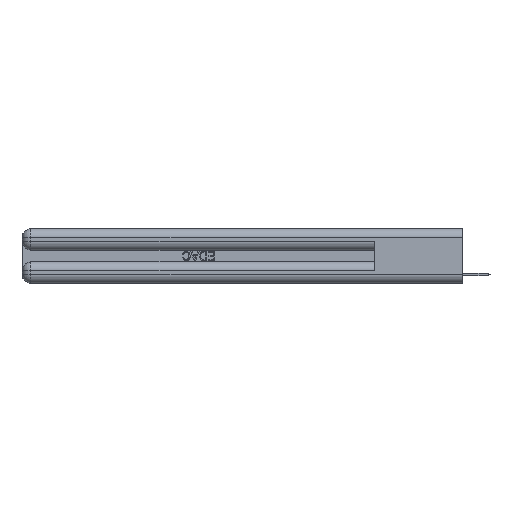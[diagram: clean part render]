
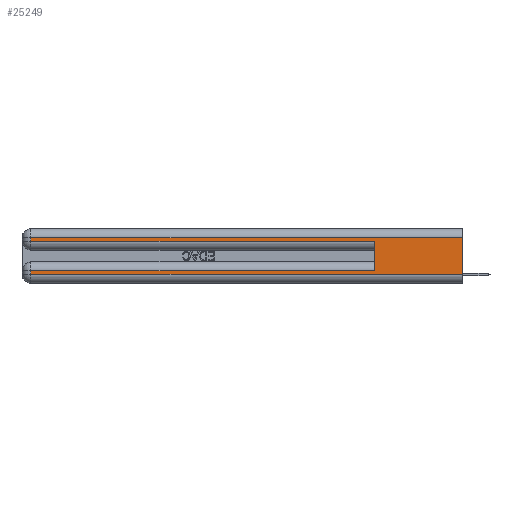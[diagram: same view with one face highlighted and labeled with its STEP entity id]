
A CAD part, left-side view. The second image highlights one B-rep face of the part: STEP entity #25249.
In plain terms, the highlighted planar face has unit normal (-1, 0, 0).
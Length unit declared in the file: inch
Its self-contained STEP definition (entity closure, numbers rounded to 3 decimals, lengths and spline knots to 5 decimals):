
#1609 = DIRECTION ( 'NONE',  ( 0., 0., -1. ) ) ;
#1629 = ORIENTED_EDGE ( 'NONE', *, *, #11532, .T. ) ;
#1727 = EDGE_CURVE ( 'NONE', #17138, #13982, #14834, .T. ) ;
#2143 = LINE ( 'NONE', #9626, #22051 ) ;
#2520 = FACE_OUTER_BOUND ( 'NONE', #8874, .T. ) ;
#2685 = DIRECTION ( 'NONE',  ( 0., 0., -1. ) ) ;
#2948 = EDGE_CURVE ( 'NONE', #13889, #15670, #12256, .T. ) ;
#3368 = AXIS2_PLACEMENT_3D ( 'NONE', #9848, #12482, #2685 ) ;
#3454 = EDGE_CURVE ( 'NONE', #17138, #5443, #7812, .T. ) ;
#3779 = LINE ( 'NONE', #6388, #30195 ) ;
#3824 = VECTOR ( 'NONE', #15304, 39.37008 ) ;
#4625 = VECTOR ( 'NONE', #1609, 39.37008 ) ;
#5028 = DIRECTION ( 'NONE',  ( 0., 1., 0. ) ) ;
#5140 = CARTESIAN_POINT ( 'NONE',  ( 0., 2.94, 0.06 ) ) ;
#5443 = VERTEX_POINT ( 'NONE', #14780 ) ;
#5764 = ORIENTED_EDGE ( 'NONE', *, *, #1727, .F. ) ;
#5929 = ORIENTED_EDGE ( 'NONE', *, *, #3454, .T. ) ;
#6388 = CARTESIAN_POINT ( 'NONE',  ( 0., 2.94, 0.37 ) ) ;
#7779 = DIRECTION ( 'NONE',  ( 0., -1., 0. ) ) ;
#7812 = LINE ( 'NONE', #18726, #26995 ) ;
#8249 = VECTOR ( 'NONE', #22666, 39.37008 ) ;
#8874 = EDGE_LOOP ( 'NONE', ( #5764, #5929, #21747, #1629, #26146, #16826, #12478, #14573 ) ) ;
#9342 = CARTESIAN_POINT ( 'NONE',  ( 0., 2.94, 0.285 ) ) ;
#9626 = CARTESIAN_POINT ( 'NONE',  ( 0., 0., 0.285 ) ) ;
#9848 = CARTESIAN_POINT ( 'NONE',  ( 0., 0., 0.37 ) ) ;
#9956 = DIRECTION ( 'NONE',  ( 0., -1., 0. ) ) ;
#10290 = CARTESIAN_POINT ( 'NONE',  ( 0., 0., 0.085 ) ) ;
#11532 = EDGE_CURVE ( 'NONE', #18070, #18893, #2143, .T. ) ;
#12256 = LINE ( 'NONE', #10290, #13425 ) ;
#12478 = ORIENTED_EDGE ( 'NONE', *, *, #17093, .T. ) ;
#12482 = DIRECTION ( 'NONE',  ( 1., 0., 0. ) ) ;
#12916 = DIRECTION ( 'NONE',  ( 0., 1., 0. ) ) ;
#13425 = VECTOR ( 'NONE', #12916, 39.37008 ) ;
#13889 = VERTEX_POINT ( 'NONE', #23014 ) ;
#13982 = VERTEX_POINT ( 'NONE', #28550 ) ;
#14223 = DIRECTION ( 'NONE',  ( 0., 0., -1. ) ) ;
#14573 = ORIENTED_EDGE ( 'NONE', *, *, #24828, .T. ) ;
#14780 = CARTESIAN_POINT ( 'NONE',  ( 0., 2.94, 0.31 ) ) ;
#14834 = LINE ( 'NONE', #20220, #8249 ) ;
#15098 = PLANE ( 'NONE',  #3368 ) ;
#15304 = DIRECTION ( 'NONE',  ( 0., 0., 1. ) ) ;
#15670 = VERTEX_POINT ( 'NONE', #23943 ) ;
#16826 = ORIENTED_EDGE ( 'NONE', *, *, #2948, .T. ) ;
#17093 = EDGE_CURVE ( 'NONE', #15670, #30240, #3779, .T. ) ;
#17138 = VERTEX_POINT ( 'NONE', #28766 ) ;
#17758 = LINE ( 'NONE', #27719, #27301 ) ;
#18070 = VERTEX_POINT ( 'NONE', #9342 ) ;
#18726 = CARTESIAN_POINT ( 'NONE',  ( 0., 0., 0.31 ) ) ;
#18893 = VERTEX_POINT ( 'NONE', #28909 ) ;
#18914 = CARTESIAN_POINT ( 'NONE',  ( 0., 2.94, 0.37 ) ) ;
#20220 = CARTESIAN_POINT ( 'NONE',  ( 0., 0., 0.37 ) ) ;
#21747 = ORIENTED_EDGE ( 'NONE', *, *, #30032, .T. ) ;
#22051 = VECTOR ( 'NONE', #9956, 39.37008 ) ;
#22087 = EDGE_CURVE ( 'NONE', #13889, #18893, #30158, .T. ) ;
#22666 = DIRECTION ( 'NONE',  ( 0., 0., -1. ) ) ;
#23014 = CARTESIAN_POINT ( 'NONE',  ( 0., 0.6, 0.085 ) ) ;
#23943 = CARTESIAN_POINT ( 'NONE',  ( 0., 2.94, 0.085 ) ) ;
#24138 = LINE ( 'NONE', #18914, #4625 ) ;
#24828 = EDGE_CURVE ( 'NONE', #30240, #13982, #17758, .T. ) ;
#25249 = ADVANCED_FACE ( 'NONE', ( #2520 ), #15098, .F. ) ;
#26146 = ORIENTED_EDGE ( 'NONE', *, *, #22087, .F. ) ;
#26995 = VECTOR ( 'NONE', #5028, 39.37008 ) ;
#27301 = VECTOR ( 'NONE', #7779, 39.37008 ) ;
#27719 = CARTESIAN_POINT ( 'NONE',  ( 0., 0., 0.06 ) ) ;
#27872 = CARTESIAN_POINT ( 'NONE',  ( 0., 0.6, 0.145 ) ) ;
#28550 = CARTESIAN_POINT ( 'NONE',  ( 0., 0., 0.06 ) ) ;
#28766 = CARTESIAN_POINT ( 'NONE',  ( 0., 0., 0.31 ) ) ;
#28909 = CARTESIAN_POINT ( 'NONE',  ( 0., 0.6, 0.285 ) ) ;
#30032 = EDGE_CURVE ( 'NONE', #5443, #18070, #24138, .T. ) ;
#30158 = LINE ( 'NONE', #27872, #3824 ) ;
#30195 = VECTOR ( 'NONE', #14223, 39.37008 ) ;
#30240 = VERTEX_POINT ( 'NONE', #5140 ) ;
